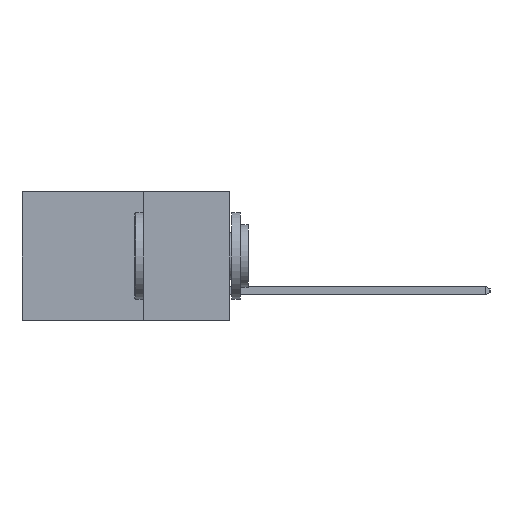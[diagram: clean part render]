
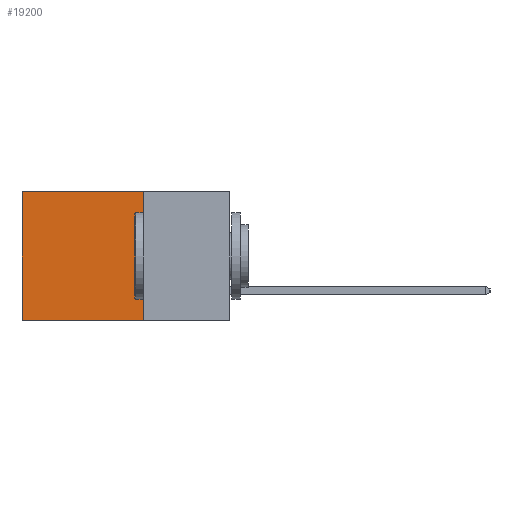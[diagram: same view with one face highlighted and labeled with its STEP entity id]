
A CAD part, left-side view. The second image highlights one B-rep face of the part: STEP entity #19200.
In plain terms, the highlighted planar face has unit normal (-1, 0, 0).
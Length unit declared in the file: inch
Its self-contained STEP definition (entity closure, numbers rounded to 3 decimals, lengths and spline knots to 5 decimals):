
#1542 = DIRECTION ( 'NONE',  ( 0., 0., -1. ) ) ;
#1783 = DIRECTION ( 'NONE',  ( 0., 0., -1. ) ) ;
#1969 = VECTOR ( 'NONE', #11276, 39.37008 ) ;
#3284 = VERTEX_POINT ( 'NONE', #18235 ) ;
#4301 = VECTOR ( 'NONE', #18922, 39.37008 ) ;
#4854 = LINE ( 'NONE', #18197, #24406 ) ;
#5171 = CARTESIAN_POINT ( 'NONE',  ( 0.2615, 0.25, 0. ) ) ;
#5584 = CARTESIAN_POINT ( 'NONE',  ( 0.2615, 0.25, -0.37 ) ) ;
#6402 = LINE ( 'NONE', #20808, #1969 ) ;
#8464 = EDGE_CURVE ( 'NONE', #17518, #3284, #16247, .T. ) ;
#9143 = CARTESIAN_POINT ( 'NONE',  ( 0.2615, 0.6, -0.37 ) ) ;
#11022 = VERTEX_POINT ( 'NONE', #18020 ) ;
#11069 = ORIENTED_EDGE ( 'NONE', *, *, #22502, .F. ) ;
#11276 = DIRECTION ( 'NONE',  ( 0., 0., -1. ) ) ;
#12767 = ORIENTED_EDGE ( 'NONE', *, *, #8464, .T. ) ;
#13136 = DIRECTION ( 'NONE',  ( 1., 0., 0. ) ) ;
#13654 = EDGE_CURVE ( 'NONE', #11022, #3284, #20085, .T. ) ;
#14084 = EDGE_CURVE ( 'NONE', #22303, #17518, #4854, .T. ) ;
#15054 = VECTOR ( 'NONE', #1542, 39.37008 ) ;
#15848 = CARTESIAN_POINT ( 'NONE',  ( 0.2615, 0.6, 0. ) ) ;
#16247 = LINE ( 'NONE', #9143, #15054 ) ;
#17518 = VERTEX_POINT ( 'NONE', #15848 ) ;
#18020 = CARTESIAN_POINT ( 'NONE',  ( 0.2615, 0.25, -0.37 ) ) ;
#18197 = CARTESIAN_POINT ( 'NONE',  ( 0.2615, 0.25, 0. ) ) ;
#18235 = CARTESIAN_POINT ( 'NONE',  ( 0.2615, 0.6, -0.37 ) ) ;
#18763 = AXIS2_PLACEMENT_3D ( 'NONE', #24428, #13136, #1783 ) ;
#18922 = DIRECTION ( 'NONE',  ( 0., 1., 0. ) ) ;
#19200 = ADVANCED_FACE ( 'NONE', ( #23710 ), #20730, .F. ) ;
#20085 = LINE ( 'NONE', #5584, #4301 ) ;
#20118 = DIRECTION ( 'NONE',  ( 0., 1., 0. ) ) ;
#20426 = EDGE_LOOP ( 'NONE', ( #12767, #23960, #11069, #20477 ) ) ;
#20477 = ORIENTED_EDGE ( 'NONE', *, *, #14084, .T. ) ;
#20730 = PLANE ( 'NONE',  #18763 ) ;
#20808 = CARTESIAN_POINT ( 'NONE',  ( 0.2615, 0.25, -0.37 ) ) ;
#22303 = VERTEX_POINT ( 'NONE', #5171 ) ;
#22502 = EDGE_CURVE ( 'NONE', #22303, #11022, #6402, .T. ) ;
#23710 = FACE_OUTER_BOUND ( 'NONE', #20426, .T. ) ;
#23960 = ORIENTED_EDGE ( 'NONE', *, *, #13654, .F. ) ;
#24406 = VECTOR ( 'NONE', #20118, 39.37008 ) ;
#24428 = CARTESIAN_POINT ( 'NONE',  ( 0.2615, 0.25, -0.37 ) ) ;
